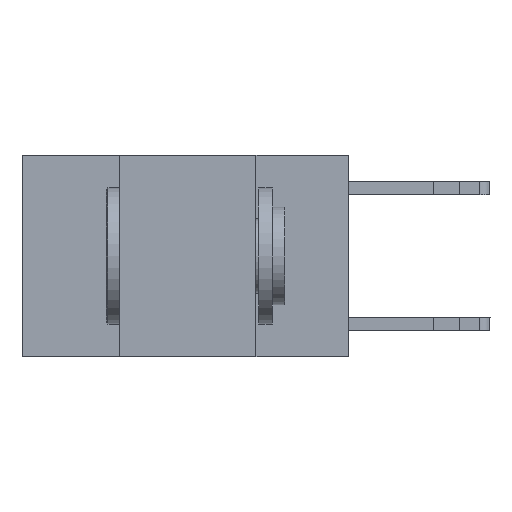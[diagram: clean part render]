
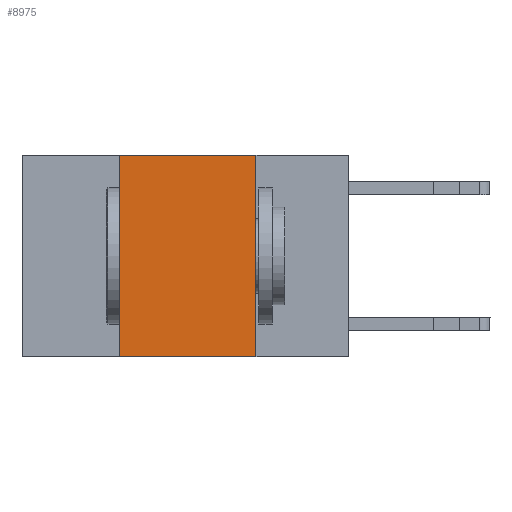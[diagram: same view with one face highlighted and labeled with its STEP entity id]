
A CAD part, left-side view. The second image highlights one B-rep face of the part: STEP entity #8975.
In plain terms, the highlighted planar face has unit normal (-1, 0, 0).
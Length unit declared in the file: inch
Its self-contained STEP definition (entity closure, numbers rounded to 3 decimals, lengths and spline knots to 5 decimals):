
#425 = DIRECTION ( 'NONE',  ( 0., 0., 1. ) ) ;
#583 = ORIENTED_EDGE ( 'NONE', *, *, #3180, .F. ) ;
#612 = VERTEX_POINT ( 'NONE', #3539 ) ;
#890 = CARTESIAN_POINT ( 'NONE',  ( 0., 0.6, 0. ) ) ;
#938 = CARTESIAN_POINT ( 'NONE',  ( 0., 0.42, 0. ) ) ;
#1512 = VECTOR ( 'NONE', #9200, 39.37008 ) ;
#2595 = VERTEX_POINT ( 'NONE', #9746 ) ;
#2746 = AXIS2_PLACEMENT_3D ( 'NONE', #890, #10380, #4775 ) ;
#3180 = EDGE_CURVE ( 'NONE', #7087, #7287, #7289, .T. ) ;
#3449 = EDGE_CURVE ( 'NONE', #2595, #612, #4073, .T. ) ;
#3469 = EDGE_CURVE ( 'NONE', #7087, #612, #11240, .T. ) ;
#3539 = CARTESIAN_POINT ( 'NONE',  ( 0., 0.17, -0.37 ) ) ;
#3833 = PLANE ( 'NONE',  #2746 ) ;
#3936 = CARTESIAN_POINT ( 'NONE',  ( 0., 0.6, -0.37 ) ) ;
#4073 = LINE ( 'NONE', #6233, #6562 ) ;
#4313 = FACE_OUTER_BOUND ( 'NONE', #5191, .T. ) ;
#4750 = DIRECTION ( 'NONE',  ( 0., 0., -1. ) ) ;
#4775 = DIRECTION ( 'NONE',  ( 0., 0., -1. ) ) ;
#5191 = EDGE_LOOP ( 'NONE', ( #6828, #11506, #583, #11778 ) ) ;
#5642 = CARTESIAN_POINT ( 'NONE',  ( 0., 0.42, -0.37 ) ) ;
#5825 = DIRECTION ( 'NONE',  ( 0., -1., 0. ) ) ;
#6102 = CARTESIAN_POINT ( 'NONE',  ( 0., 0.42, 0. ) ) ;
#6233 = CARTESIAN_POINT ( 'NONE',  ( 0., 0.17, 0. ) ) ;
#6562 = VECTOR ( 'NONE', #4750, 39.37008 ) ;
#6828 = ORIENTED_EDGE ( 'NONE', *, *, #3449, .F. ) ;
#7087 = VERTEX_POINT ( 'NONE', #5642 ) ;
#7287 = VERTEX_POINT ( 'NONE', #6102 ) ;
#7289 = LINE ( 'NONE', #938, #9193 ) ;
#7374 = LINE ( 'NONE', #10474, #12047 ) ;
#8411 = EDGE_CURVE ( 'NONE', #7287, #2595, #7374, .T. ) ;
#8975 = ADVANCED_FACE ( 'NONE', ( #4313 ), #3833, .F. ) ;
#9193 = VECTOR ( 'NONE', #425, 39.37008 ) ;
#9200 = DIRECTION ( 'NONE',  ( 0., -1., 0. ) ) ;
#9746 = CARTESIAN_POINT ( 'NONE',  ( 0., 0.17, 0. ) ) ;
#10380 = DIRECTION ( 'NONE',  ( 1., 0., 0. ) ) ;
#10474 = CARTESIAN_POINT ( 'NONE',  ( 0., 0.6, 0. ) ) ;
#11240 = LINE ( 'NONE', #3936, #1512 ) ;
#11506 = ORIENTED_EDGE ( 'NONE', *, *, #8411, .F. ) ;
#11778 = ORIENTED_EDGE ( 'NONE', *, *, #3469, .T. ) ;
#12047 = VECTOR ( 'NONE', #5825, 39.37008 ) ;
